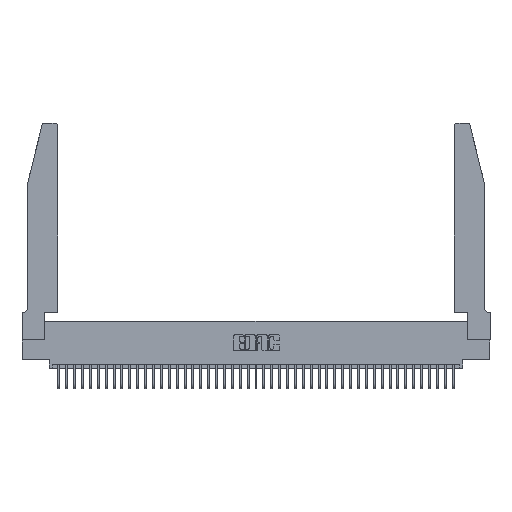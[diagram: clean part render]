
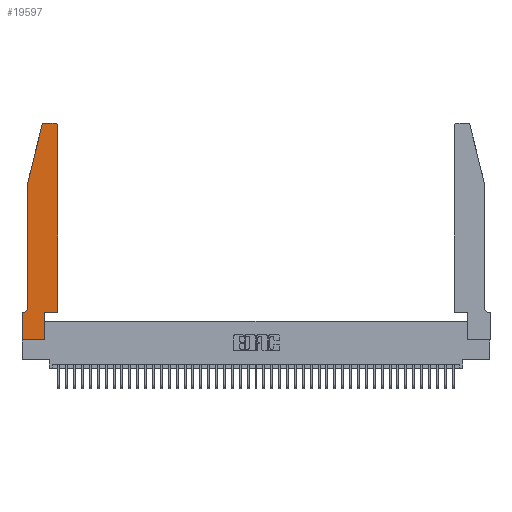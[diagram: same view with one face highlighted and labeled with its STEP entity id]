
A CAD part, top view. The second image highlights one B-rep face of the part: STEP entity #19597.
In plain terms, the highlighted planar face has unit normal (0, 0, 1).
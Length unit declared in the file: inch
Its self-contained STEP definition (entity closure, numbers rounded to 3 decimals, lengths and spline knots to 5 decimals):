
#79 = LINE ( 'NONE', #33777, #16462 ) ;
#207 = DIRECTION ( 'NONE',  ( 0., 1., 0. ) ) ;
#221 = AXIS2_PLACEMENT_3D ( 'NONE', #37525, #18140, #40791 ) ;
#454 = EDGE_CURVE ( 'NONE', #40155, #17160, #32006, .T. ) ;
#1073 = CARTESIAN_POINT ( 'NONE',  ( 0., 0., 0.37 ) ) ;
#1189 = ORIENTED_EDGE ( 'NONE', *, *, #32272, .T. ) ;
#1215 = CARTESIAN_POINT ( 'NONE',  ( 0., 0.35, 0.37 ) ) ;
#1887 = DIRECTION ( 'NONE',  ( -1., 0., 0. ) ) ;
#1920 = DIRECTION ( 'NONE',  ( -1., 0., 0. ) ) ;
#2078 = FACE_OUTER_BOUND ( 'NONE', #31490, .T. ) ;
#2085 = CARTESIAN_POINT ( 'NONE',  ( 0.25487, 2.72718, 0.37 ) ) ;
#2129 = VERTEX_POINT ( 'NONE', #2085 ) ;
#2165 = EDGE_CURVE ( 'NONE', #38652, #41314, #17367, .T. ) ;
#2447 = VERTEX_POINT ( 'NONE', #7083 ) ;
#2745 = ORIENTED_EDGE ( 'NONE', *, *, #38810, .T. ) ;
#3359 = CARTESIAN_POINT ( 'NONE',  ( 0.2865, 0.35, 0.37 ) ) ;
#4438 = VECTOR ( 'NONE', #32756, 39.37008 ) ;
#4769 = VERTEX_POINT ( 'NONE', #26509 ) ;
#6016 = LINE ( 'NONE', #11915, #38544 ) ;
#6223 = CIRCLE ( 'NONE', #221, 0.03 ) ;
#6369 = ORIENTED_EDGE ( 'NONE', *, *, #2165, .T. ) ;
#6407 = AXIS2_PLACEMENT_3D ( 'NONE', #10443, #33123, #13686 ) ;
#7083 = CARTESIAN_POINT ( 'NONE',  ( 0.4505, 2.72, 0.37 ) ) ;
#7177 = EDGE_CURVE ( 'NONE', #36241, #4769, #79, .T. ) ;
#7382 = LINE ( 'NONE', #17166, #40894 ) ;
#7929 = DIRECTION ( 'NONE',  ( 1., 0., 0. ) ) ;
#9381 = CARTESIAN_POINT ( 'NONE',  ( 0.4505, 0.35, 0.37 ) ) ;
#9584 = ORIENTED_EDGE ( 'NONE', *, *, #18378, .T. ) ;
#9666 = CARTESIAN_POINT ( 'NONE',  ( 0.4205, 2.75, 0.37 ) ) ;
#9805 = CARTESIAN_POINT ( 'NONE',  ( 0.2865, 0., 0.37 ) ) ;
#10081 = CARTESIAN_POINT ( 'NONE',  ( 0., 0., 0.37 ) ) ;
#10364 = AXIS2_PLACEMENT_3D ( 'NONE', #18781, #41466, #22031 ) ;
#10443 = CARTESIAN_POINT ( 'NONE',  ( 0.284, 2.72, 0.37 ) ) ;
#11441 = ORIENTED_EDGE ( 'NONE', *, *, #30400, .T. ) ;
#11915 = CARTESIAN_POINT ( 'NONE',  ( 0., 0., 0.37 ) ) ;
#12134 = LINE ( 'NONE', #10081, #4438 ) ;
#12630 = DIRECTION ( 'NONE',  ( 0., 1., 0. ) ) ;
#13012 = VECTOR ( 'NONE', #17313, 39.37008 ) ;
#13686 = DIRECTION ( 'NONE',  ( 1., 0., 0. ) ) ;
#14350 = PLANE ( 'NONE',  #23975 ) ;
#14430 = LINE ( 'NONE', #14922, #36232 ) ;
#14922 = CARTESIAN_POINT ( 'NONE',  ( 0.0755, 0.35, 0.37 ) ) ;
#15128 = EDGE_CURVE ( 'NONE', #41983, #40467, #6016, .T. ) ;
#15417 = EDGE_CURVE ( 'NONE', #25736, #41983, #12134, .T. ) ;
#15642 = CARTESIAN_POINT ( 'NONE',  ( 0.4505, 0.35, 0.37 ) ) ;
#15961 = DIRECTION ( 'NONE',  ( 1., 0., 0. ) ) ;
#16462 = VECTOR ( 'NONE', #1920, 39.37008 ) ;
#16953 = VECTOR ( 'NONE', #12630, 39.37008 ) ;
#17160 = VERTEX_POINT ( 'NONE', #15642 ) ;
#17166 = CARTESIAN_POINT ( 'NONE',  ( 0.0755, 2., 0.37 ) ) ;
#17313 = DIRECTION ( 'NONE',  ( 0., -1., 0. ) ) ;
#17367 = CIRCLE ( 'NONE', #10364, 0.07 ) ;
#18140 = DIRECTION ( 'NONE',  ( 0., 0., 1. ) ) ;
#18153 = CARTESIAN_POINT ( 'NONE',  ( 0.2865, 0.35, 0.37 ) ) ;
#18378 = EDGE_CURVE ( 'NONE', #2447, #36241, #6223, .T. ) ;
#18781 = CARTESIAN_POINT ( 'NONE',  ( 0.0055, 0.42, 0.37 ) ) ;
#19597 = ADVANCED_FACE ( 'NONE', ( #2078 ), #14350, .T. ) ;
#20195 = EDGE_CURVE ( 'NONE', #17160, #2447, #25551, .T. ) ;
#21696 = VECTOR ( 'NONE', #207, 39.37008 ) ;
#22031 = DIRECTION ( 'NONE',  ( -1., 0., 0. ) ) ;
#23487 = CARTESIAN_POINT ( 'NONE',  ( 0.0055, 0.35, 0.37 ) ) ;
#23975 = AXIS2_PLACEMENT_3D ( 'NONE', #24097, #27388, #7929 ) ;
#24097 = CARTESIAN_POINT ( 'NONE',  ( 0., 0.35, 0.37 ) ) ;
#24643 = ORIENTED_EDGE ( 'NONE', *, *, #7177, .T. ) ;
#25208 = ORIENTED_EDGE ( 'NONE', *, *, #38179, .T. ) ;
#25551 = LINE ( 'NONE', #9381, #16953 ) ;
#25722 = CARTESIAN_POINT ( 'NONE',  ( 0.4505, 0.35, 0.37 ) ) ;
#25736 = VERTEX_POINT ( 'NONE', #1215 ) ;
#25800 = ORIENTED_EDGE ( 'NONE', *, *, #20195, .T. ) ;
#25917 = CARTESIAN_POINT ( 'NONE',  ( 0.0755, 0.42, 0.37 ) ) ;
#26236 = ORIENTED_EDGE ( 'NONE', *, *, #15417, .T. ) ;
#26509 = CARTESIAN_POINT ( 'NONE',  ( 0.284, 2.75, 0.37 ) ) ;
#27128 = VERTEX_POINT ( 'NONE', #37353 ) ;
#27388 = DIRECTION ( 'NONE',  ( 0., 0., 1. ) ) ;
#28099 = DIRECTION ( 'NONE',  ( 1., 0., 0. ) ) ;
#29582 = EDGE_CURVE ( 'NONE', #40467, #40155, #30336, .T. ) ;
#30243 = CIRCLE ( 'NONE', #6407, 0.03 ) ;
#30336 = LINE ( 'NONE', #3359, #21696 ) ;
#30400 = EDGE_CURVE ( 'NONE', #2129, #27128, #7382, .T. ) ;
#31490 = EDGE_LOOP ( 'NONE', ( #24643, #2745, #11441, #25208, #6369, #1189, #26236, #35477, #38856, #31897, #25800, #9584 ) ) ;
#31897 = ORIENTED_EDGE ( 'NONE', *, *, #454, .T. ) ;
#32006 = LINE ( 'NONE', #25722, #38591 ) ;
#32272 = EDGE_CURVE ( 'NONE', #41314, #25736, #14430, .T. ) ;
#32756 = DIRECTION ( 'NONE',  ( 0., -1., 0. ) ) ;
#33123 = DIRECTION ( 'NONE',  ( 0., 0., 1. ) ) ;
#33444 = CARTESIAN_POINT ( 'NONE',  ( 0.0755, 2., 0.37 ) ) ;
#33777 = CARTESIAN_POINT ( 'NONE',  ( 0.2605, 2.75, 0.37 ) ) ;
#35477 = ORIENTED_EDGE ( 'NONE', *, *, #15128, .T. ) ;
#36232 = VECTOR ( 'NONE', #1887, 39.37008 ) ;
#36241 = VERTEX_POINT ( 'NONE', #9666 ) ;
#36561 = DIRECTION ( 'NONE',  ( -0.239, -0.971, 0. ) ) ;
#37353 = CARTESIAN_POINT ( 'NONE',  ( 0.0755, 2., 0.37 ) ) ;
#37525 = CARTESIAN_POINT ( 'NONE',  ( 0.4205, 2.72, 0.37 ) ) ;
#38179 = EDGE_CURVE ( 'NONE', #27128, #38652, #38917, .T. ) ;
#38544 = VECTOR ( 'NONE', #28099, 39.37008 ) ;
#38591 = VECTOR ( 'NONE', #15961, 39.37008 ) ;
#38652 = VERTEX_POINT ( 'NONE', #25917 ) ;
#38810 = EDGE_CURVE ( 'NONE', #4769, #2129, #30243, .T. ) ;
#38856 = ORIENTED_EDGE ( 'NONE', *, *, #29582, .T. ) ;
#38917 = LINE ( 'NONE', #33444, #13012 ) ;
#40155 = VERTEX_POINT ( 'NONE', #18153 ) ;
#40467 = VERTEX_POINT ( 'NONE', #9805 ) ;
#40791 = DIRECTION ( 'NONE',  ( 1., 0., 0. ) ) ;
#40894 = VECTOR ( 'NONE', #36561, 39.37008 ) ;
#41314 = VERTEX_POINT ( 'NONE', #23487 ) ;
#41466 = DIRECTION ( 'NONE',  ( 0., 0., -1. ) ) ;
#41983 = VERTEX_POINT ( 'NONE', #1073 ) ;
